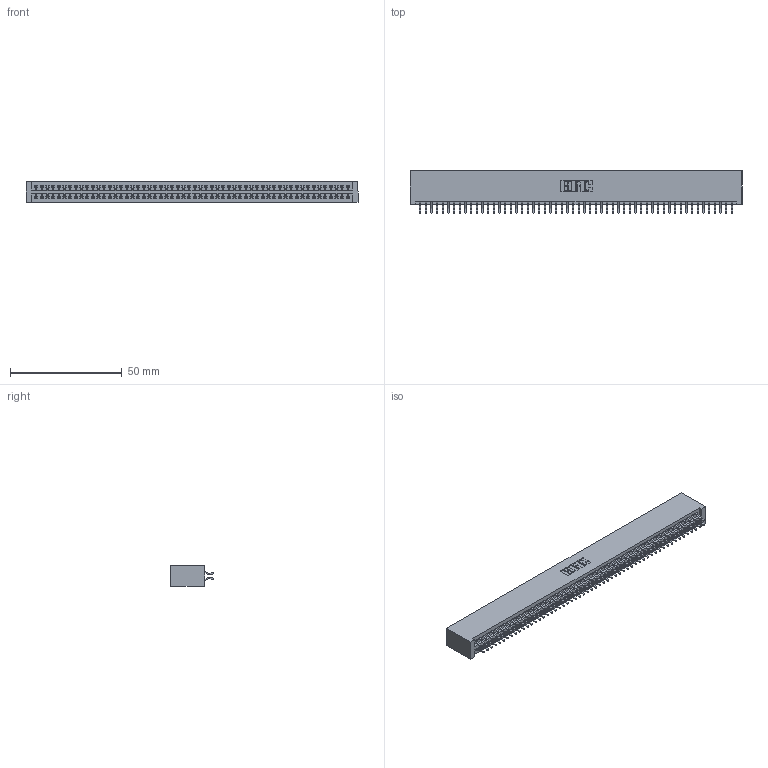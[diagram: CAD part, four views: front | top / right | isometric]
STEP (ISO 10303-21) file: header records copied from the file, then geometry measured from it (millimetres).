
FILE_DESCRIPTION (( 'STEP AP203' ), '1' );
FILE_NAME ('395-112-556-201.STEP', '2019-10-27T16:01:59', ( '' ), ( '' ), 'SwSTEP 2.0', 'SolidWorks 2016', '' );
FILE_SCHEMA (( 'CONFIG_CONTROL_DESIGN' ));
Length unit declared in the file: inch
Products named in the file (3): 345 Part_No Mounting Lugs; 345-292-001_556 Tail; 395-112-556-201
Assembly tree (113 placements, depth 2):
  395-112-556-201
    345 Part_No Mounting Lugs
    345-292-001_556 Tail  x112
Bounding box: 148.84 x 19.24 x 9.4 mm (x, y, z)
Volume: 15200.3 mm3; surface area: 22945 mm2
Topology: 113 solids, 113 shells, 6390 faces, 19021 edges, 12530 vertices
Faces by surface type: plane 4220, cylinder 2170
Entity records: 41997 total; most frequent: CARTESIAN_POINT 7040, ORIENTED_EDGE 6962, DIRECTION 6173, EDGE_CURVE 3481, VECTOR 3125, LINE 3125, VERTEX_POINT 2318, AXIS2_PLACEMENT_3D 1524
